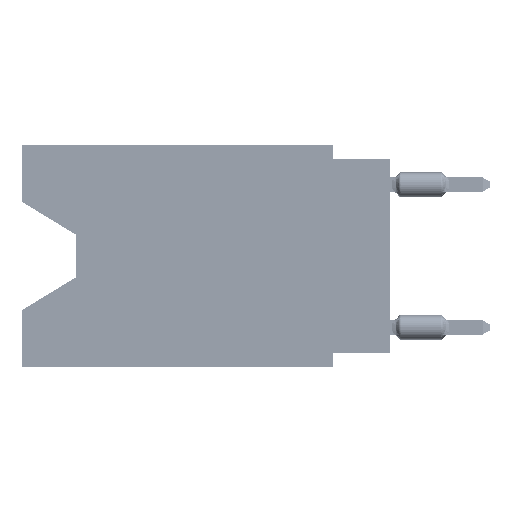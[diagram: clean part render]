
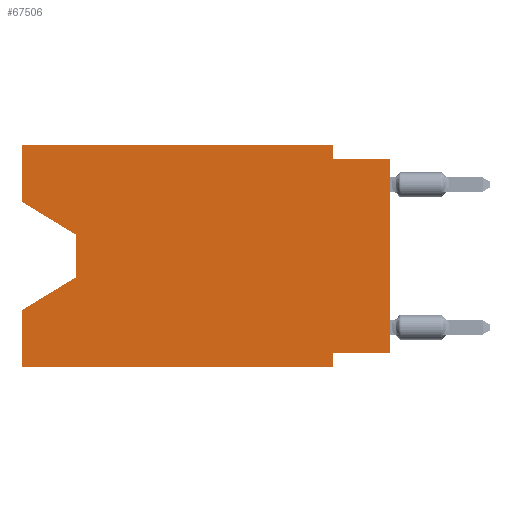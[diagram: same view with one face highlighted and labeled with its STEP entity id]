
A CAD part, left-side view. The second image highlights one B-rep face of the part: STEP entity #67506.
In plain terms, the highlighted planar face has unit normal (-1, 0, 0).
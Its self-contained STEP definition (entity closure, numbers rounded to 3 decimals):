
#246 = LINE ( 'NONE', #68432, #7256 ) ;
#410 = CARTESIAN_POINT ( 'NONE',  ( 0., 16.383, -7.36 ) ) ;
#797 = EDGE_CURVE ( 'NONE', #9566, #3833, #20741, .T. ) ;
#1378 = VECTOR ( 'NONE', #46306, 1000. ) ;
#1703 = DIRECTION ( 'NONE',  ( 1., 0., 0. ) ) ;
#3218 = CARTESIAN_POINT ( 'NONE',  ( 0., 13.97, -5.893 ) ) ;
#3717 = VERTEX_POINT ( 'NONE', #6690 ) ;
#3833 = VERTEX_POINT ( 'NONE', #25959 ) ;
#4949 = DIRECTION ( 'NONE',  ( 0., -1., 0. ) ) ;
#5151 = CARTESIAN_POINT ( 'NONE',  ( 0., 0., 0. ) ) ;
#5635 = VECTOR ( 'NONE', #42579, 1000. ) ;
#6690 = CARTESIAN_POINT ( 'NONE',  ( 0., 16.383, -9.906 ) ) ;
#7004 = DIRECTION ( 'NONE',  ( 0., -0.855, -0.519 ) ) ;
#7256 = VECTOR ( 'NONE', #33183, 1000. ) ;
#7379 = PLANE ( 'NONE',  #44123 ) ;
#7393 = EDGE_CURVE ( 'NONE', #28976, #64392, #24042, .T. ) ;
#7785 = EDGE_CURVE ( 'NONE', #3833, #29225, #58078, .T. ) ;
#8572 = EDGE_CURVE ( 'NONE', #74318, #57083, #46033, .T. ) ;
#9403 = DIRECTION ( 'NONE',  ( 0., 1., 0. ) ) ;
#9566 = VERTEX_POINT ( 'NONE', #59488 ) ;
#10715 = LINE ( 'NONE', #61481, #17404 ) ;
#12921 = EDGE_CURVE ( 'NONE', #3717, #66542, #19118, .T. ) ;
#14393 = CARTESIAN_POINT ( 'NONE',  ( 0., 2.54, 0. ) ) ;
#14736 = CARTESIAN_POINT ( 'NONE',  ( 0., 2.54, -0.635 ) ) ;
#14972 = LINE ( 'NONE', #3218, #5635 ) ;
#15470 = CARTESIAN_POINT ( 'NONE',  ( 0., 13.97, -5.893 ) ) ;
#17404 = VECTOR ( 'NONE', #32648, 1000. ) ;
#17435 = EDGE_LOOP ( 'NONE', ( #19867, #69697, #49395, #26043, #31935, #33892, #58203, #60733, #20693, #50575, #42876, #60394 ) ) ;
#18743 = CARTESIAN_POINT ( 'NONE',  ( 0., 16.383, 0. ) ) ;
#19118 = LINE ( 'NONE', #65323, #51211 ) ;
#19284 = VERTEX_POINT ( 'NONE', #37885 ) ;
#19867 = ORIENTED_EDGE ( 'NONE', *, *, #7393, .T. ) ;
#20693 = ORIENTED_EDGE ( 'NONE', *, *, #8572, .F. ) ;
#20741 = LINE ( 'NONE', #62036, #58756 ) ;
#21570 = EDGE_CURVE ( 'NONE', #64392, #31420, #246, .T. ) ;
#23439 = CARTESIAN_POINT ( 'NONE',  ( 0., 2.54, -9.906 ) ) ;
#23709 = VECTOR ( 'NONE', #37128, 1000. ) ;
#23876 = EDGE_CURVE ( 'NONE', #27808, #74318, #28596, .T. ) ;
#24042 = LINE ( 'NONE', #58907, #44868 ) ;
#25959 = CARTESIAN_POINT ( 'NONE',  ( 0., 2.54, -9.271 ) ) ;
#26043 = ORIENTED_EDGE ( 'NONE', *, *, #12921, .F. ) ;
#26693 = EDGE_CURVE ( 'NONE', #9566, #57083, #67274, .T. ) ;
#27663 = CARTESIAN_POINT ( 'NONE',  ( 0., 16.383, 0. ) ) ;
#27808 = VERTEX_POINT ( 'NONE', #14393 ) ;
#28596 = LINE ( 'NONE', #74803, #42526 ) ;
#28976 = VERTEX_POINT ( 'NONE', #48837 ) ;
#28987 = FACE_OUTER_BOUND ( 'NONE', #17435, .T. ) ;
#29225 = VERTEX_POINT ( 'NONE', #23439 ) ;
#29316 = VECTOR ( 'NONE', #58928, 1000. ) ;
#30097 = CARTESIAN_POINT ( 'NONE',  ( 0., 0., -0.635 ) ) ;
#31420 = VERTEX_POINT ( 'NONE', #15470 ) ;
#31935 = ORIENTED_EDGE ( 'NONE', *, *, #48147, .T. ) ;
#32615 = EDGE_CURVE ( 'NONE', #28976, #19284, #47754, .T. ) ;
#32648 = DIRECTION ( 'NONE',  ( 0., -1., 0. ) ) ;
#32790 = EDGE_CURVE ( 'NONE', #19284, #27808, #45448, .T. ) ;
#33183 = DIRECTION ( 'NONE',  ( 0., 0., -1. ) ) ;
#33892 = ORIENTED_EDGE ( 'NONE', *, *, #7785, .F. ) ;
#34151 = VECTOR ( 'NONE', #73692, 1000. ) ;
#34867 = CARTESIAN_POINT ( 'NONE',  ( 0., 13.97, -4.013 ) ) ;
#37128 = DIRECTION ( 'NONE',  ( 0., 0., 1. ) ) ;
#37885 = CARTESIAN_POINT ( 'NONE',  ( 0., 16.383, 0. ) ) ;
#42526 = VECTOR ( 'NONE', #45993, 1000. ) ;
#42579 = DIRECTION ( 'NONE',  ( 0., 0.855, -0.519 ) ) ;
#42876 = ORIENTED_EDGE ( 'NONE', *, *, #32790, .F. ) ;
#44123 = AXIS2_PLACEMENT_3D ( 'NONE', #18743, #1703, #64951 ) ;
#44868 = VECTOR ( 'NONE', #7004, 1000. ) ;
#45448 = LINE ( 'NONE', #27663, #49097 ) ;
#45993 = DIRECTION ( 'NONE',  ( 0., 0., -1. ) ) ;
#46033 = LINE ( 'NONE', #30097, #29316 ) ;
#46306 = DIRECTION ( 'NONE',  ( 0., 0., -1. ) ) ;
#47754 = LINE ( 'NONE', #53819, #23709 ) ;
#48147 = EDGE_CURVE ( 'NONE', #3717, #29225, #10715, .T. ) ;
#48837 = CARTESIAN_POINT ( 'NONE',  ( 0., 16.383, -2.546 ) ) ;
#49097 = VECTOR ( 'NONE', #4949, 1000. ) ;
#49395 = ORIENTED_EDGE ( 'NONE', *, *, #68819, .T. ) ;
#50575 = ORIENTED_EDGE ( 'NONE', *, *, #23876, .F. ) ;
#51211 = VECTOR ( 'NONE', #60411, 1000. ) ;
#53819 = CARTESIAN_POINT ( 'NONE',  ( 0., 16.383, 0. ) ) ;
#57083 = VERTEX_POINT ( 'NONE', #57438 ) ;
#57438 = CARTESIAN_POINT ( 'NONE',  ( 0., 0., -0.635 ) ) ;
#58078 = LINE ( 'NONE', #64115, #1378 ) ;
#58203 = ORIENTED_EDGE ( 'NONE', *, *, #797, .F. ) ;
#58756 = VECTOR ( 'NONE', #9403, 1000. ) ;
#58907 = CARTESIAN_POINT ( 'NONE',  ( 0., 16.383, -2.546 ) ) ;
#58928 = DIRECTION ( 'NONE',  ( 0., -1., 0. ) ) ;
#59488 = CARTESIAN_POINT ( 'NONE',  ( 0., 0., -9.271 ) ) ;
#60394 = ORIENTED_EDGE ( 'NONE', *, *, #32615, .F. ) ;
#60411 = DIRECTION ( 'NONE',  ( 0., 0., 1. ) ) ;
#60733 = ORIENTED_EDGE ( 'NONE', *, *, #26693, .T. ) ;
#61481 = CARTESIAN_POINT ( 'NONE',  ( 0., 16.383, -9.906 ) ) ;
#62036 = CARTESIAN_POINT ( 'NONE',  ( 0., 0., -9.271 ) ) ;
#64115 = CARTESIAN_POINT ( 'NONE',  ( 0., 2.54, -9.906 ) ) ;
#64392 = VERTEX_POINT ( 'NONE', #34867 ) ;
#64951 = DIRECTION ( 'NONE',  ( 0., 0., -1. ) ) ;
#65323 = CARTESIAN_POINT ( 'NONE',  ( 0., 16.383, 0. ) ) ;
#66542 = VERTEX_POINT ( 'NONE', #410 ) ;
#67274 = LINE ( 'NONE', #5151, #34151 ) ;
#67506 = ADVANCED_FACE ( 'NONE', ( #28987 ), #7379, .F. ) ;
#68432 = CARTESIAN_POINT ( 'NONE',  ( 0., 13.97, -4.013 ) ) ;
#68819 = EDGE_CURVE ( 'NONE', #31420, #66542, #14972, .T. ) ;
#69697 = ORIENTED_EDGE ( 'NONE', *, *, #21570, .T. ) ;
#73692 = DIRECTION ( 'NONE',  ( 0., 0., 1. ) ) ;
#74318 = VERTEX_POINT ( 'NONE', #14736 ) ;
#74803 = CARTESIAN_POINT ( 'NONE',  ( 0., 2.54, 0. ) ) ;
